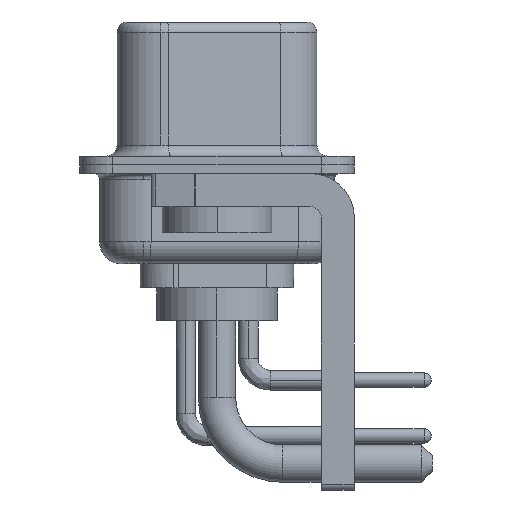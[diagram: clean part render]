
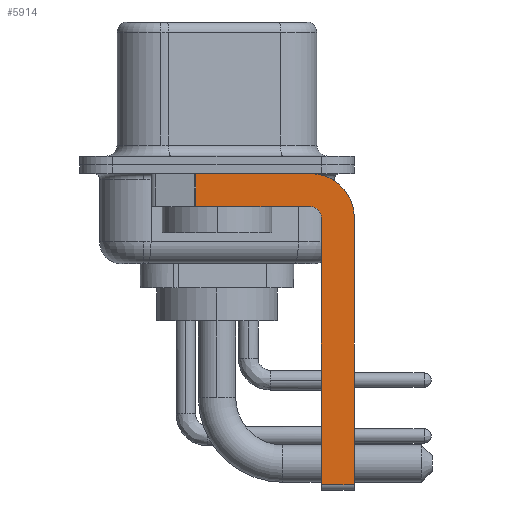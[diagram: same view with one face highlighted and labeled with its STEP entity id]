
A CAD part, left-side view. The second image highlights one B-rep face of the part: STEP entity #5914.
In plain terms, the highlighted planar face has unit normal (-1, 0, 0).
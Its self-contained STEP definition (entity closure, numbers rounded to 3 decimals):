
#17 = CARTESIAN_POINT ( 'NONE',  ( -2.9, -4.25, -1.9 ) ) ;
#574 = VERTEX_POINT ( 'NONE', #16646 ) ;
#636 = VECTOR ( 'NONE', #21953, 1000. ) ;
#857 = CARTESIAN_POINT ( 'NONE',  ( -2.9, 0.978, -1.9 ) ) ;
#1491 = CIRCLE ( 'NONE', #16008, 0.5 ) ;
#2123 = VERTEX_POINT ( 'NONE', #24956 ) ;
#3043 = FACE_OUTER_BOUND ( 'NONE', #17155, .T. ) ;
#3235 = DIRECTION ( 'NONE',  ( 0., 0., -1. ) ) ;
#4248 = EDGE_CURVE ( 'NONE', #15069, #19006, #16312, .T. ) ;
#5124 = CARTESIAN_POINT ( 'NONE',  ( -2.9, -4.25, -2.4 ) ) ;
#5201 = EDGE_CURVE ( 'NONE', #23314, #2123, #5378, .T. ) ;
#5250 = VERTEX_POINT ( 'NONE', #13303 ) ;
#5341 = VECTOR ( 'NONE', #8795, 1000. ) ;
#5378 = LINE ( 'NONE', #18392, #5380 ) ;
#5380 = VECTOR ( 'NONE', #23164, 1000. ) ;
#5388 = EDGE_CURVE ( 'NONE', #15069, #5250, #25371, .T. ) ;
#5478 = EDGE_CURVE ( 'NONE', #9542, #7466, #6262, .T. ) ;
#5808 = VECTOR ( 'NONE', #9536, 1000. ) ;
#5914 = ADVANCED_FACE ( 'NONE', ( #3043 ), #9410, .F. ) ;
#6229 = DIRECTION ( 'NONE',  ( -1., 0., 0. ) ) ;
#6262 = LINE ( 'NONE', #21971, #19913 ) ;
#6619 = CARTESIAN_POINT ( 'NONE',  ( -2.9, -4.25, -2.4 ) ) ;
#6980 = ORIENTED_EDGE ( 'NONE', *, *, #9607, .F. ) ;
#7381 = DIRECTION ( 'NONE',  ( 0., -1., 0. ) ) ;
#7466 = VERTEX_POINT ( 'NONE', #7713 ) ;
#7713 = CARTESIAN_POINT ( 'NONE',  ( -2.9, -4.75, -2.4 ) ) ;
#8231 = EDGE_CURVE ( 'NONE', #5250, #23314, #21156, .T. ) ;
#8795 = DIRECTION ( 'NONE',  ( 0., 0., -1. ) ) ;
#9146 = AXIS2_PLACEMENT_3D ( 'NONE', #15057, #25054, #3235 ) ;
#9159 = ORIENTED_EDGE ( 'NONE', *, *, #23788, .F. ) ;
#9410 = PLANE ( 'NONE',  #23665 ) ;
#9536 = DIRECTION ( 'NONE',  ( 0., -1., 0. ) ) ;
#9542 = VERTEX_POINT ( 'NONE', #10127 ) ;
#9607 = EDGE_CURVE ( 'NONE', #574, #19006, #19753, .T. ) ;
#10102 = CARTESIAN_POINT ( 'NONE',  ( -2.9, 0.978, -1.9 ) ) ;
#10127 = CARTESIAN_POINT ( 'NONE',  ( -2.9, -4.75, -14.55 ) ) ;
#10587 = ORIENTED_EDGE ( 'NONE', *, *, #5478, .F. ) ;
#10823 = ORIENTED_EDGE ( 'NONE', *, *, #11344, .T. ) ;
#11272 = CARTESIAN_POINT ( 'NONE',  ( -2.9, -4.25, -14.55 ) ) ;
#11344 = EDGE_CURVE ( 'NONE', #9542, #2123, #21274, .T. ) ;
#11663 = ORIENTED_EDGE ( 'NONE', *, *, #8231, .F. ) ;
#12085 = ORIENTED_EDGE ( 'NONE', *, *, #4248, .T. ) ;
#12254 = ORIENTED_EDGE ( 'NONE', *, *, #5201, .F. ) ;
#12493 = DIRECTION ( 'NONE',  ( 0., 0., 1. ) ) ;
#12619 = CARTESIAN_POINT ( 'NONE',  ( -2.9, -6.25, -2.4 ) ) ;
#13303 = CARTESIAN_POINT ( 'NONE',  ( -2.9, -4.25, -0.4 ) ) ;
#15057 = CARTESIAN_POINT ( 'NONE',  ( -2.9, -4.25, -2.4 ) ) ;
#15069 = VERTEX_POINT ( 'NONE', #22441 ) ;
#16008 = AXIS2_PLACEMENT_3D ( 'NONE', #6619, #6229, #16096 ) ;
#16096 = DIRECTION ( 'NONE',  ( 0., 0., 1. ) ) ;
#16312 = LINE ( 'NONE', #857, #5341 ) ;
#16646 = CARTESIAN_POINT ( 'NONE',  ( -2.9, -4.25, -1.9 ) ) ;
#17155 = EDGE_LOOP ( 'NONE', ( #25696, #12085, #6980, #9159, #10587, #10823, #12254, #11663 ) ) ;
#18392 = CARTESIAN_POINT ( 'NONE',  ( -2.9, -6.25, -2.4 ) ) ;
#18884 = DIRECTION ( 'NONE',  ( 1., 0., 0. ) ) ;
#19006 = VERTEX_POINT ( 'NONE', #10102 ) ;
#19753 = LINE ( 'NONE', #17, #636 ) ;
#19913 = VECTOR ( 'NONE', #12493, 1000. ) ;
#21104 = DIRECTION ( 'NONE',  ( 0., 0., -1. ) ) ;
#21156 = CIRCLE ( 'NONE', #9146, 2. ) ;
#21274 = LINE ( 'NONE', #11272, #25378 ) ;
#21953 = DIRECTION ( 'NONE',  ( 0., 1., 0. ) ) ;
#21971 = CARTESIAN_POINT ( 'NONE',  ( -2.9, -4.75, -14.8 ) ) ;
#22441 = CARTESIAN_POINT ( 'NONE',  ( -2.9, 0.978, -0.4 ) ) ;
#23164 = DIRECTION ( 'NONE',  ( 0., 0., -1. ) ) ;
#23314 = VERTEX_POINT ( 'NONE', #12619 ) ;
#23665 = AXIS2_PLACEMENT_3D ( 'NONE', #5124, #18884, #21104 ) ;
#23788 = EDGE_CURVE ( 'NONE', #7466, #574, #1491, .T. ) ;
#24956 = CARTESIAN_POINT ( 'NONE',  ( -2.9, -6.25, -14.55 ) ) ;
#25054 = DIRECTION ( 'NONE',  ( 1., 0., 0. ) ) ;
#25371 = LINE ( 'NONE', #25492, #5808 ) ;
#25378 = VECTOR ( 'NONE', #7381, 1000. ) ;
#25492 = CARTESIAN_POINT ( 'NONE',  ( -2.9, 3., -0.4 ) ) ;
#25696 = ORIENTED_EDGE ( 'NONE', *, *, #5388, .F. ) ;
